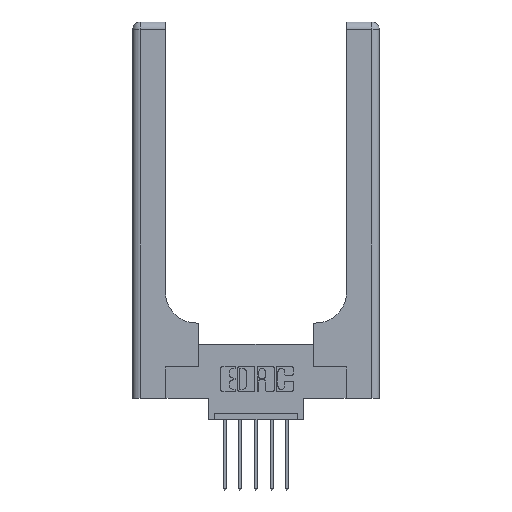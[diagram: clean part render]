
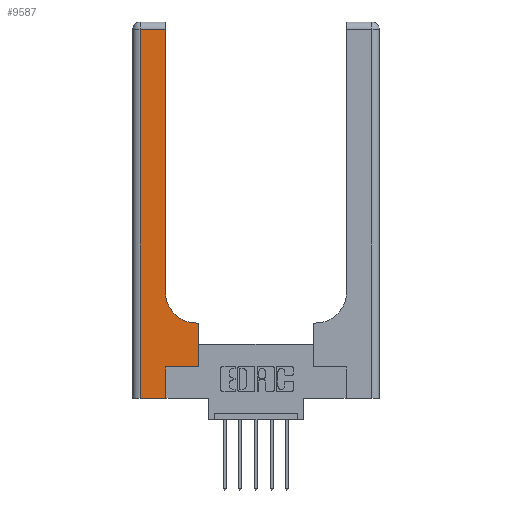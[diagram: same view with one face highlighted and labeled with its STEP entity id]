
A CAD part, top view. The second image highlights one B-rep face of the part: STEP entity #9587.
In plain terms, the highlighted planar face has unit normal (0, 0, 1).
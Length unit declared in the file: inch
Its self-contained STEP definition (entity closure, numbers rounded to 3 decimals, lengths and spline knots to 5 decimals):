
#35 = LINE ( 'NONE', #878, #6893 ) ;
#128 = EDGE_CURVE ( 'NONE', #13607, #4363, #9664, .T. ) ;
#523 = ORIENTED_EDGE ( 'NONE', *, *, #13716, .T. ) ;
#662 = EDGE_CURVE ( 'NONE', #5618, #7944, #1157, .T. ) ;
#757 = CARTESIAN_POINT ( 'NONE',  ( 0., 0., 0.37 ) ) ;
#772 = AXIS2_PLACEMENT_3D ( 'NONE', #6094, #10107, #8076 ) ;
#878 = CARTESIAN_POINT ( 'NONE',  ( 0.528, 0.25, 0.37 ) ) ;
#898 = ORIENTED_EDGE ( 'NONE', *, *, #1829, .T. ) ;
#1022 = DIRECTION ( 'NONE',  ( -1., 0., 0. ) ) ;
#1082 = DIRECTION ( 'NONE',  ( 0., 1., 0. ) ) ;
#1157 = LINE ( 'NONE', #4374, #10111 ) ;
#1829 = EDGE_CURVE ( 'NONE', #7944, #13607, #11881, .T. ) ;
#2136 = CARTESIAN_POINT ( 'NONE',  ( 0., 3., 0.37 ) ) ;
#2276 = DIRECTION ( 'NONE',  ( -1., 0., 0. ) ) ;
#2594 = EDGE_CURVE ( 'NONE', #4363, #2883, #13300, .T. ) ;
#2883 = VERTEX_POINT ( 'NONE', #11138 ) ;
#2909 = CARTESIAN_POINT ( 'NONE',  ( 0.265, 0.25, 0.37 ) ) ;
#3111 = ORIENTED_EDGE ( 'NONE', *, *, #2594, .T. ) ;
#3352 = CARTESIAN_POINT ( 'NONE',  ( 0.26, 0.6, 0.37 ) ) ;
#3798 = CARTESIAN_POINT ( 'NONE',  ( 0.528, 0.25, 0.37 ) ) ;
#4222 = ORIENTED_EDGE ( 'NONE', *, *, #10967, .T. ) ;
#4363 = VERTEX_POINT ( 'NONE', #12254 ) ;
#4374 = CARTESIAN_POINT ( 'NONE',  ( 0.26, 3., 0.37 ) ) ;
#4595 = VECTOR ( 'NONE', #12609, 39.37008 ) ;
#4672 = CARTESIAN_POINT ( 'NONE',  ( 0.26, 0.85, 0.37 ) ) ;
#5046 = EDGE_CURVE ( 'NONE', #6983, #5773, #35, .T. ) ;
#5176 = CARTESIAN_POINT ( 'NONE',  ( 0.06, 3., 0.37 ) ) ;
#5243 = DIRECTION ( 'NONE',  ( 0., -1., 0. ) ) ;
#5298 = PLANE ( 'NONE',  #10364 ) ;
#5312 = CARTESIAN_POINT ( 'NONE',  ( 0.528, 0.6, 0.37 ) ) ;
#5452 = EDGE_CURVE ( 'NONE', #5773, #7806, #8762, .T. ) ;
#5490 = DIRECTION ( 'NONE',  ( 0., 1., 0. ) ) ;
#5618 = VERTEX_POINT ( 'NONE', #4672 ) ;
#5773 = VERTEX_POINT ( 'NONE', #5312 ) ;
#6094 = CARTESIAN_POINT ( 'NONE',  ( 0.51, 0.85, 0.37 ) ) ;
#6173 = DIRECTION ( 'NONE',  ( 0., 1., 0. ) ) ;
#6893 = VECTOR ( 'NONE', #1082, 39.37008 ) ;
#6983 = VERTEX_POINT ( 'NONE', #3798 ) ;
#7029 = CIRCLE ( 'NONE', #772, 0.25 ) ;
#7082 = VECTOR ( 'NONE', #6173, 39.37008 ) ;
#7369 = VECTOR ( 'NONE', #7640, 39.37008 ) ;
#7400 = DIRECTION ( 'NONE',  ( 0., 0., -1. ) ) ;
#7640 = DIRECTION ( 'NONE',  ( -1., 0., 0. ) ) ;
#7806 = VERTEX_POINT ( 'NONE', #11478 ) ;
#7944 = VERTEX_POINT ( 'NONE', #11761 ) ;
#8076 = DIRECTION ( 'NONE',  ( 1., 0., 0. ) ) ;
#8199 = VECTOR ( 'NONE', #2276, 39.37008 ) ;
#8254 = VERTEX_POINT ( 'NONE', #2909 ) ;
#8337 = LINE ( 'NONE', #11702, #4595 ) ;
#8762 = LINE ( 'NONE', #3352, #7369 ) ;
#8797 = CARTESIAN_POINT ( 'NONE',  ( 0., 2.94, 0.37 ) ) ;
#8808 = ORIENTED_EDGE ( 'NONE', *, *, #5046, .T. ) ;
#8955 = ORIENTED_EDGE ( 'NONE', *, *, #12664, .T. ) ;
#9551 = VECTOR ( 'NONE', #13232, 39.37008 ) ;
#9587 = ADVANCED_FACE ( 'NONE', ( #13783 ), #5298, .F. ) ;
#9664 = LINE ( 'NONE', #5176, #11116 ) ;
#10107 = DIRECTION ( 'NONE',  ( 0., 0., -1. ) ) ;
#10111 = VECTOR ( 'NONE', #5490, 39.37008 ) ;
#10114 = CARTESIAN_POINT ( 'NONE',  ( 0.06, 2.94, 0.37 ) ) ;
#10364 = AXIS2_PLACEMENT_3D ( 'NONE', #2136, #7400, #1022 ) ;
#10448 = EDGE_LOOP ( 'NONE', ( #12755, #898, #11898, #3111, #523, #8955, #8808, #11932, #4222 ) ) ;
#10462 = LINE ( 'NONE', #11580, #7082 ) ;
#10967 = EDGE_CURVE ( 'NONE', #7806, #5618, #7029, .T. ) ;
#11116 = VECTOR ( 'NONE', #5243, 39.37008 ) ;
#11138 = CARTESIAN_POINT ( 'NONE',  ( 0.265, 0., 0.37 ) ) ;
#11478 = CARTESIAN_POINT ( 'NONE',  ( 0.51, 0.6, 0.37 ) ) ;
#11580 = CARTESIAN_POINT ( 'NONE',  ( 0.265, 0., 0.37 ) ) ;
#11702 = CARTESIAN_POINT ( 'NONE',  ( 0.265, 0.25, 0.37 ) ) ;
#11761 = CARTESIAN_POINT ( 'NONE',  ( 0.26, 2.94, 0.37 ) ) ;
#11881 = LINE ( 'NONE', #8797, #8199 ) ;
#11898 = ORIENTED_EDGE ( 'NONE', *, *, #128, .T. ) ;
#11932 = ORIENTED_EDGE ( 'NONE', *, *, #5452, .T. ) ;
#12254 = CARTESIAN_POINT ( 'NONE',  ( 0.06, 0., 0.37 ) ) ;
#12609 = DIRECTION ( 'NONE',  ( 1., 0., 0. ) ) ;
#12664 = EDGE_CURVE ( 'NONE', #8254, #6983, #8337, .T. ) ;
#12755 = ORIENTED_EDGE ( 'NONE', *, *, #662, .T. ) ;
#13232 = DIRECTION ( 'NONE',  ( 1., 0., 0. ) ) ;
#13300 = LINE ( 'NONE', #757, #9551 ) ;
#13607 = VERTEX_POINT ( 'NONE', #10114 ) ;
#13716 = EDGE_CURVE ( 'NONE', #2883, #8254, #10462, .T. ) ;
#13783 = FACE_OUTER_BOUND ( 'NONE', #10448, .T. ) ;
